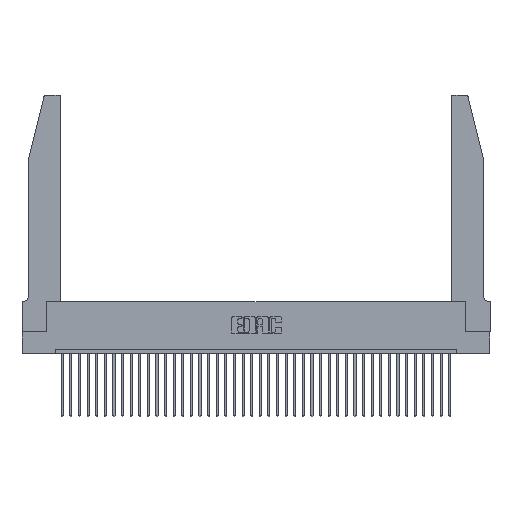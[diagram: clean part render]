
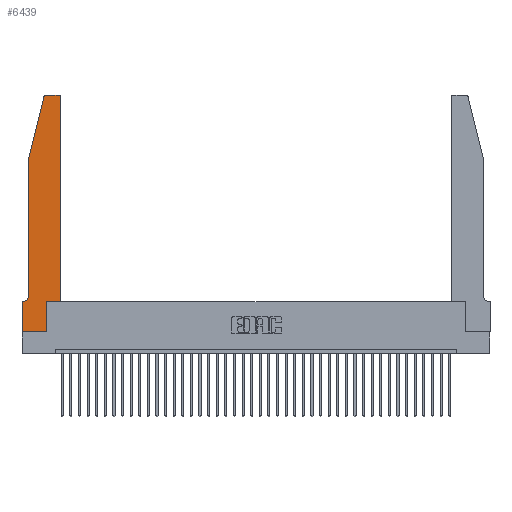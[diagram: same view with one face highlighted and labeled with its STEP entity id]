
A CAD part, top view. The second image highlights one B-rep face of the part: STEP entity #6439.
In plain terms, the highlighted planar face has unit normal (0, 0, 1).
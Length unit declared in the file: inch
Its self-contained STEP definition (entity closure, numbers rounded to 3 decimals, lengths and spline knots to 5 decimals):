
#364 = EDGE_CURVE ( 'NONE', #1748, #9295, #15894, .T. ) ;
#792 = DIRECTION ( 'NONE',  ( 1., 0., 0. ) ) ;
#891 = CARTESIAN_POINT ( 'NONE',  ( 0.4505, 2.72, 0.37 ) ) ;
#1280 = CARTESIAN_POINT ( 'NONE',  ( 0.4205, 2.75, 0.37 ) ) ;
#1748 = VERTEX_POINT ( 'NONE', #12040 ) ;
#1879 = DIRECTION ( 'NONE',  ( -0.239, -0.971, 0. ) ) ;
#2232 = EDGE_CURVE ( 'NONE', #3310, #31030, #37843, .T. ) ;
#2963 = CARTESIAN_POINT ( 'NONE',  ( 0., 0., 0.37 ) ) ;
#3082 = DIRECTION ( 'NONE',  ( -1., 0., 0. ) ) ;
#3310 = VERTEX_POINT ( 'NONE', #891 ) ;
#3314 = DIRECTION ( 'NONE',  ( 1., 0., 0. ) ) ;
#3520 = FACE_OUTER_BOUND ( 'NONE', #17327, .T. ) ;
#3701 = CARTESIAN_POINT ( 'NONE',  ( 0.2865, 0.35, 0.37 ) ) ;
#3936 = LINE ( 'NONE', #7537, #38232 ) ;
#3994 = CARTESIAN_POINT ( 'NONE',  ( 0., 0.35, 0.37 ) ) ;
#4275 = DIRECTION ( 'NONE',  ( 0., 0., 1. ) ) ;
#4323 = DIRECTION ( 'NONE',  ( 0., -1., 0. ) ) ;
#4552 = CARTESIAN_POINT ( 'NONE',  ( 0.284, 2.72, 0.37 ) ) ;
#4772 = ORIENTED_EDGE ( 'NONE', *, *, #2232, .T. ) ;
#5029 = ORIENTED_EDGE ( 'NONE', *, *, #37947, .T. ) ;
#6439 = ADVANCED_FACE ( 'NONE', ( #3520 ), #16060, .T. ) ;
#6601 = LINE ( 'NONE', #13154, #13693 ) ;
#7537 = CARTESIAN_POINT ( 'NONE',  ( 0.4505, 0.35, 0.37 ) ) ;
#7684 = CARTESIAN_POINT ( 'NONE',  ( 0., 0., 0.37 ) ) ;
#7966 = AXIS2_PLACEMENT_3D ( 'NONE', #8827, #36026, #11990 ) ;
#8785 = EDGE_CURVE ( 'NONE', #30147, #9738, #19357, .T. ) ;
#8827 = CARTESIAN_POINT ( 'NONE',  ( 0.0055, 0.42, 0.37 ) ) ;
#9122 = ORIENTED_EDGE ( 'NONE', *, *, #31958, .T. ) ;
#9167 = CIRCLE ( 'NONE', #17553, 0.03 ) ;
#9295 = VERTEX_POINT ( 'NONE', #9937 ) ;
#9629 = DIRECTION ( 'NONE',  ( 1., 0., 0. ) ) ;
#9738 = VERTEX_POINT ( 'NONE', #23318 ) ;
#9818 = LINE ( 'NONE', #35937, #20655 ) ;
#9890 = EDGE_CURVE ( 'NONE', #21128, #23570, #9818, .T. ) ;
#9937 = CARTESIAN_POINT ( 'NONE',  ( 0.2865, 0.35, 0.37 ) ) ;
#10340 = LINE ( 'NONE', #17648, #30045 ) ;
#11629 = ORIENTED_EDGE ( 'NONE', *, *, #34425, .T. ) ;
#11990 = DIRECTION ( 'NONE',  ( -1., 0., 0. ) ) ;
#12040 = CARTESIAN_POINT ( 'NONE',  ( 0.2865, 0., 0.37 ) ) ;
#12127 = CARTESIAN_POINT ( 'NONE',  ( 0.0755, 2., 0.37 ) ) ;
#12583 = CARTESIAN_POINT ( 'NONE',  ( 0.4205, 2.72, 0.37 ) ) ;
#13154 = CARTESIAN_POINT ( 'NONE',  ( 0.2605, 2.75, 0.37 ) ) ;
#13693 = VECTOR ( 'NONE', #34094, 39.37008 ) ;
#15271 = ORIENTED_EDGE ( 'NONE', *, *, #9890, .T. ) ;
#15894 = LINE ( 'NONE', #3701, #37015 ) ;
#15908 = VECTOR ( 'NONE', #1879, 39.37008 ) ;
#16060 = PLANE ( 'NONE',  #28355 ) ;
#16571 = ORIENTED_EDGE ( 'NONE', *, *, #23002, .T. ) ;
#16826 = CARTESIAN_POINT ( 'NONE',  ( 0.0755, 2., 0.37 ) ) ;
#17175 = VECTOR ( 'NONE', #29919, 39.37008 ) ;
#17327 = EDGE_LOOP ( 'NONE', ( #30440, #11629, #31642, #29608, #23362, #15271, #9122, #29558, #21167, #16571, #5029, #4772 ) ) ;
#17553 = AXIS2_PLACEMENT_3D ( 'NONE', #4552, #4275, #25264 ) ;
#17648 = CARTESIAN_POINT ( 'NONE',  ( 0., 0., 0.37 ) ) ;
#19357 = LINE ( 'NONE', #22410, #33350 ) ;
#20072 = CARTESIAN_POINT ( 'NONE',  ( 0.0055, 0.35, 0.37 ) ) ;
#20655 = VECTOR ( 'NONE', #3082, 39.37008 ) ;
#21128 = VERTEX_POINT ( 'NONE', #20072 ) ;
#21167 = ORIENTED_EDGE ( 'NONE', *, *, #364, .T. ) ;
#22410 = CARTESIAN_POINT ( 'NONE',  ( 0.0755, 2., 0.37 ) ) ;
#23002 = EDGE_CURVE ( 'NONE', #9295, #33435, #3936, .T. ) ;
#23318 = CARTESIAN_POINT ( 'NONE',  ( 0.0755, 0.42, 0.37 ) ) ;
#23362 = ORIENTED_EDGE ( 'NONE', *, *, #32712, .T. ) ;
#23570 = VERTEX_POINT ( 'NONE', #3994 ) ;
#25102 = EDGE_CURVE ( 'NONE', #29396, #1748, #34716, .T. ) ;
#25144 = DIRECTION ( 'NONE',  ( 0., 0., 1. ) ) ;
#25264 = DIRECTION ( 'NONE',  ( 1., 0., 0. ) ) ;
#25659 = VERTEX_POINT ( 'NONE', #31355 ) ;
#26048 = AXIS2_PLACEMENT_3D ( 'NONE', #12583, #31987, #792 ) ;
#26809 = CARTESIAN_POINT ( 'NONE',  ( 0.4505, 0.35, 0.37 ) ) ;
#28355 = AXIS2_PLACEMENT_3D ( 'NONE', #33728, #25144, #9629 ) ;
#29396 = VERTEX_POINT ( 'NONE', #7684 ) ;
#29558 = ORIENTED_EDGE ( 'NONE', *, *, #25102, .T. ) ;
#29608 = ORIENTED_EDGE ( 'NONE', *, *, #8785, .T. ) ;
#29838 = DIRECTION ( 'NONE',  ( 0., -1., 0. ) ) ;
#29919 = DIRECTION ( 'NONE',  ( 0., 1., 0. ) ) ;
#30045 = VECTOR ( 'NONE', #29838, 39.37008 ) ;
#30147 = VERTEX_POINT ( 'NONE', #12127 ) ;
#30423 = CIRCLE ( 'NONE', #7966, 0.07 ) ;
#30436 = EDGE_CURVE ( 'NONE', #31030, #32156, #6601, .T. ) ;
#30440 = ORIENTED_EDGE ( 'NONE', *, *, #30436, .T. ) ;
#31030 = VERTEX_POINT ( 'NONE', #1280 ) ;
#31355 = CARTESIAN_POINT ( 'NONE',  ( 0.25487, 2.72718, 0.37 ) ) ;
#31642 = ORIENTED_EDGE ( 'NONE', *, *, #32351, .T. ) ;
#31684 = LINE ( 'NONE', #26809, #17175 ) ;
#31958 = EDGE_CURVE ( 'NONE', #23570, #29396, #10340, .T. ) ;
#31987 = DIRECTION ( 'NONE',  ( 0., 0., 1. ) ) ;
#32156 = VERTEX_POINT ( 'NONE', #36309 ) ;
#32351 = EDGE_CURVE ( 'NONE', #25659, #30147, #32814, .T. ) ;
#32712 = EDGE_CURVE ( 'NONE', #9738, #21128, #30423, .T. ) ;
#32814 = LINE ( 'NONE', #16826, #15908 ) ;
#32825 = VECTOR ( 'NONE', #3314, 39.37008 ) ;
#33350 = VECTOR ( 'NONE', #4323, 39.37008 ) ;
#33435 = VERTEX_POINT ( 'NONE', #36012 ) ;
#33728 = CARTESIAN_POINT ( 'NONE',  ( 0., 0.35, 0.37 ) ) ;
#34094 = DIRECTION ( 'NONE',  ( -1., 0., 0. ) ) ;
#34425 = EDGE_CURVE ( 'NONE', #32156, #25659, #9167, .T. ) ;
#34552 = DIRECTION ( 'NONE',  ( 1., 0., 0. ) ) ;
#34716 = LINE ( 'NONE', #2963, #32825 ) ;
#35937 = CARTESIAN_POINT ( 'NONE',  ( 0.0755, 0.35, 0.37 ) ) ;
#36012 = CARTESIAN_POINT ( 'NONE',  ( 0.4505, 0.35, 0.37 ) ) ;
#36026 = DIRECTION ( 'NONE',  ( 0., 0., -1. ) ) ;
#36309 = CARTESIAN_POINT ( 'NONE',  ( 0.284, 2.75, 0.37 ) ) ;
#36709 = DIRECTION ( 'NONE',  ( 0., 1., 0. ) ) ;
#37015 = VECTOR ( 'NONE', #36709, 39.37008 ) ;
#37843 = CIRCLE ( 'NONE', #26048, 0.03 ) ;
#37947 = EDGE_CURVE ( 'NONE', #33435, #3310, #31684, .T. ) ;
#38232 = VECTOR ( 'NONE', #34552, 39.37008 ) ;
